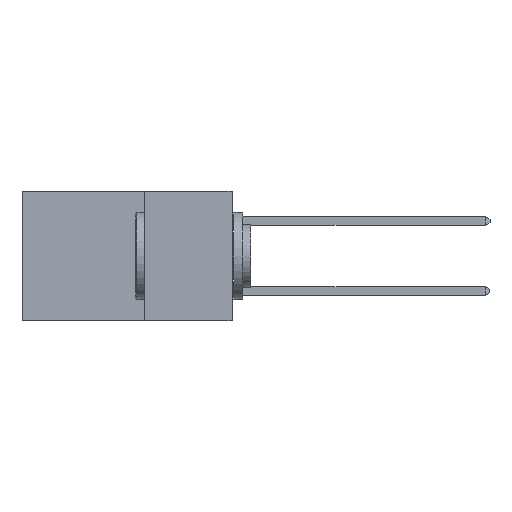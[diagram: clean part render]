
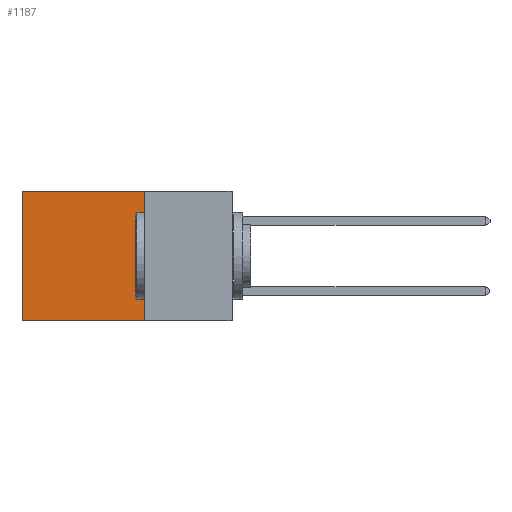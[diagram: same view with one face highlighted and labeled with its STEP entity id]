
A CAD part, left-side view. The second image highlights one B-rep face of the part: STEP entity #1187.
In plain terms, the highlighted planar face has unit normal (-1, 0, 0).
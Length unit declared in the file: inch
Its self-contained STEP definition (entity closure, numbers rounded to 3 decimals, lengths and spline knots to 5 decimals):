
#335 = ORIENTED_EDGE ( 'NONE', *, *, #3936, .T. ) ;
#692 = CARTESIAN_POINT ( 'NONE',  ( 0.2875, 0.25, 0. ) ) ;
#1121 = DIRECTION ( 'NONE',  ( 0., 1., 0. ) ) ;
#1187 = ADVANCED_FACE ( 'NONE', ( #3380 ), #12684, .F. ) ;
#1274 = CARTESIAN_POINT ( 'NONE',  ( 0.2875, 0.25, 0. ) ) ;
#1919 = DIRECTION ( 'NONE',  ( 0., 0., -1. ) ) ;
#1976 = CARTESIAN_POINT ( 'NONE',  ( 0.2875, 0.25, 0. ) ) ;
#2304 = VERTEX_POINT ( 'NONE', #11009 ) ;
#2367 = DIRECTION ( 'NONE',  ( 0., 1., 0. ) ) ;
#2886 = EDGE_CURVE ( 'NONE', #2304, #10303, #11219, .T. ) ;
#2892 = VECTOR ( 'NONE', #1919, 39.37008 ) ;
#3380 = FACE_OUTER_BOUND ( 'NONE', #11095, .T. ) ;
#3936 = EDGE_CURVE ( 'NONE', #7285, #2304, #8279, .T. ) ;
#4994 = VECTOR ( 'NONE', #1121, 39.37008 ) ;
#5773 = EDGE_CURVE ( 'NONE', #7285, #11042, #8778, .T. ) ;
#6106 = DIRECTION ( 'NONE',  ( 0., 0., -1. ) ) ;
#6296 = AXIS2_PLACEMENT_3D ( 'NONE', #12935, #12560, #12580 ) ;
#6301 = CARTESIAN_POINT ( 'NONE',  ( 0.2875, 0.6, 0. ) ) ;
#7285 = VERTEX_POINT ( 'NONE', #692 ) ;
#7497 = ORIENTED_EDGE ( 'NONE', *, *, #2886, .T. ) ;
#8087 = EDGE_CURVE ( 'NONE', #11042, #10303, #10248, .T. ) ;
#8279 = LINE ( 'NONE', #1274, #4994 ) ;
#8313 = VECTOR ( 'NONE', #6106, 39.37008 ) ;
#8778 = LINE ( 'NONE', #1976, #2892 ) ;
#10101 = ORIENTED_EDGE ( 'NONE', *, *, #5773, .F. ) ;
#10139 = CARTESIAN_POINT ( 'NONE',  ( 0.2875, 0.25, -0.37 ) ) ;
#10248 = LINE ( 'NONE', #10139, #12743 ) ;
#10303 = VERTEX_POINT ( 'NONE', #11708 ) ;
#11009 = CARTESIAN_POINT ( 'NONE',  ( 0.2875, 0.6, 0. ) ) ;
#11042 = VERTEX_POINT ( 'NONE', #11923 ) ;
#11095 = EDGE_LOOP ( 'NONE', ( #7497, #12027, #10101, #335 ) ) ;
#11219 = LINE ( 'NONE', #6301, #8313 ) ;
#11708 = CARTESIAN_POINT ( 'NONE',  ( 0.2875, 0.6, -0.37 ) ) ;
#11923 = CARTESIAN_POINT ( 'NONE',  ( 0.2875, 0.25, -0.37 ) ) ;
#12027 = ORIENTED_EDGE ( 'NONE', *, *, #8087, .F. ) ;
#12560 = DIRECTION ( 'NONE',  ( 1., 0., 0. ) ) ;
#12580 = DIRECTION ( 'NONE',  ( 0., 0., -1. ) ) ;
#12684 = PLANE ( 'NONE',  #6296 ) ;
#12743 = VECTOR ( 'NONE', #2367, 39.37008 ) ;
#12935 = CARTESIAN_POINT ( 'NONE',  ( 0.2875, 0.25, 0. ) ) ;
